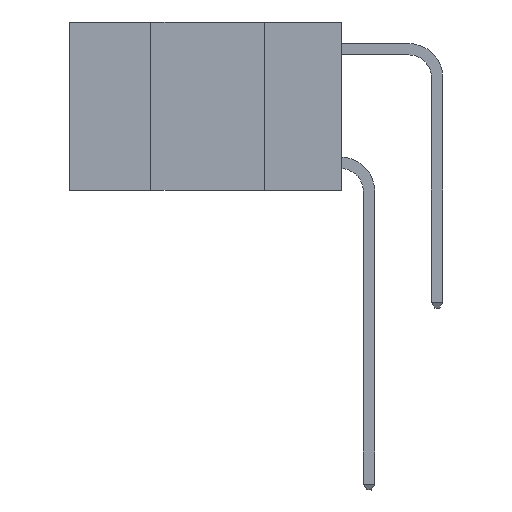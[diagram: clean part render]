
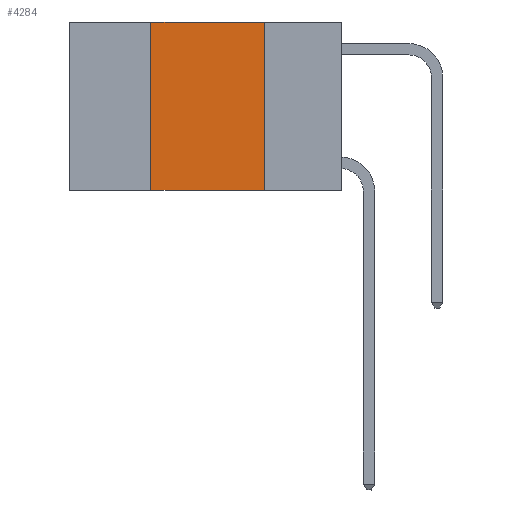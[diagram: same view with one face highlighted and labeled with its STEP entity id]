
A CAD part, left-side view. The second image highlights one B-rep face of the part: STEP entity #4284.
In plain terms, the highlighted planar face has unit normal (-1, 0, 0).
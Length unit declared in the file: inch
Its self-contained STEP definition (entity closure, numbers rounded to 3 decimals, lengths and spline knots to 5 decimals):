
#5 = CARTESIAN_POINT ( 'NONE',  ( 0., 0.6, -0.37 ) ) ;
#672 = VECTOR ( 'NONE', #12102, 39.37008 ) ;
#760 = CARTESIAN_POINT ( 'NONE',  ( 0., 0.42, 0. ) ) ;
#779 = EDGE_CURVE ( 'NONE', #11823, #10746, #8757, .T. ) ;
#1077 = VECTOR ( 'NONE', #18557, 39.37008 ) ;
#2635 = ORIENTED_EDGE ( 'NONE', *, *, #5701, .F. ) ;
#2834 = DIRECTION ( 'NONE',  ( 1., 0., 0. ) ) ;
#3112 = VECTOR ( 'NONE', #6769, 39.37008 ) ;
#3573 = LINE ( 'NONE', #16767, #3112 ) ;
#3617 = CARTESIAN_POINT ( 'NONE',  ( 0., 0.17, 0. ) ) ;
#3958 = FACE_OUTER_BOUND ( 'NONE', #5880, .T. ) ;
#4113 = LINE ( 'NONE', #3617, #672 ) ;
#4284 = ADVANCED_FACE ( 'NONE', ( #3958 ), #11380, .F. ) ;
#5601 = CARTESIAN_POINT ( 'NONE',  ( 0., 0.17, 0. ) ) ;
#5701 = EDGE_CURVE ( 'NONE', #10746, #7567, #4113, .T. ) ;
#5880 = EDGE_LOOP ( 'NONE', ( #2635, #10222, #6857, #10689 ) ) ;
#6769 = DIRECTION ( 'NONE',  ( 0., 0., 1. ) ) ;
#6857 = ORIENTED_EDGE ( 'NONE', *, *, #11283, .F. ) ;
#7567 = VERTEX_POINT ( 'NONE', #16390 ) ;
#8757 = LINE ( 'NONE', #10493, #1077 ) ;
#9165 = EDGE_CURVE ( 'NONE', #16825, #7567, #9918, .T. ) ;
#9918 = LINE ( 'NONE', #5, #17040 ) ;
#10222 = ORIENTED_EDGE ( 'NONE', *, *, #779, .F. ) ;
#10493 = CARTESIAN_POINT ( 'NONE',  ( 0., 0.6, 0. ) ) ;
#10689 = ORIENTED_EDGE ( 'NONE', *, *, #9165, .T. ) ;
#10746 = VERTEX_POINT ( 'NONE', #5601 ) ;
#11283 = EDGE_CURVE ( 'NONE', #16825, #11823, #3573, .T. ) ;
#11380 = PLANE ( 'NONE',  #11527 ) ;
#11499 = DIRECTION ( 'NONE',  ( 0., -1., 0. ) ) ;
#11527 = AXIS2_PLACEMENT_3D ( 'NONE', #17053, #2834, #12843 ) ;
#11823 = VERTEX_POINT ( 'NONE', #760 ) ;
#12102 = DIRECTION ( 'NONE',  ( 0., 0., -1. ) ) ;
#12843 = DIRECTION ( 'NONE',  ( 0., 0., -1. ) ) ;
#16390 = CARTESIAN_POINT ( 'NONE',  ( 0., 0.17, -0.37 ) ) ;
#16767 = CARTESIAN_POINT ( 'NONE',  ( 0., 0.42, 0. ) ) ;
#16825 = VERTEX_POINT ( 'NONE', #18173 ) ;
#17040 = VECTOR ( 'NONE', #11499, 39.37008 ) ;
#17053 = CARTESIAN_POINT ( 'NONE',  ( 0., 0.6, 0. ) ) ;
#18173 = CARTESIAN_POINT ( 'NONE',  ( 0., 0.42, -0.37 ) ) ;
#18557 = DIRECTION ( 'NONE',  ( 0., -1., 0. ) ) ;
